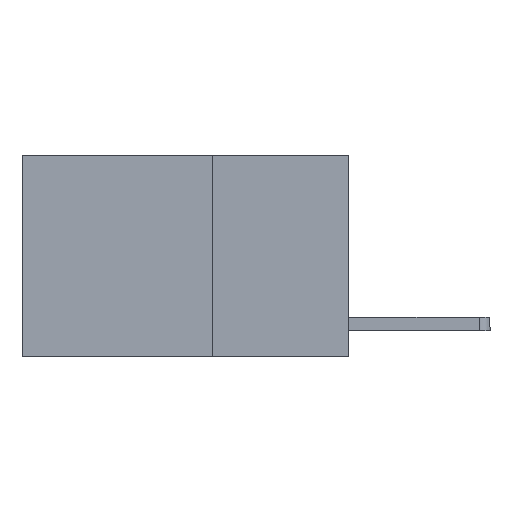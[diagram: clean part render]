
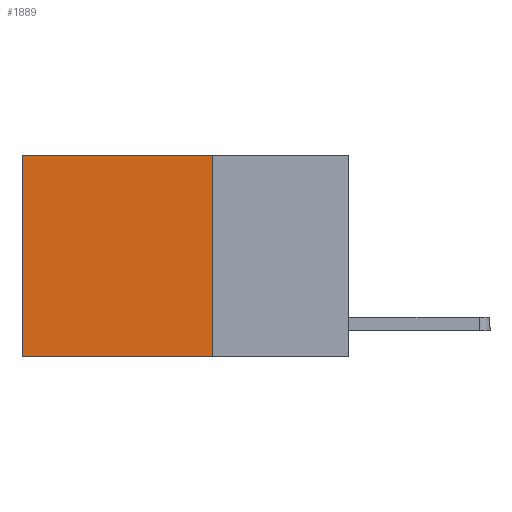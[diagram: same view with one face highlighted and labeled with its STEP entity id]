
A CAD part, left-side view. The second image highlights one B-rep face of the part: STEP entity #1889.
In plain terms, the highlighted planar face has unit normal (-1, 0, 0).
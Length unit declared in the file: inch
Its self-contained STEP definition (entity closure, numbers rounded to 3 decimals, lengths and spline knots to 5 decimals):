
#607 = LINE ( 'NONE', #1943, #8104 ) ;
#856 = VECTOR ( 'NONE', #2397, 39.37008 ) ;
#1255 = CARTESIAN_POINT ( 'NONE',  ( 0.2625, 0.25, 0. ) ) ;
#1321 = EDGE_CURVE ( 'NONE', #7605, #7886, #1727, .T. ) ;
#1387 = EDGE_LOOP ( 'NONE', ( #6431, #4426, #2238, #6048 ) ) ;
#1727 = LINE ( 'NONE', #5034, #7196 ) ;
#1889 = ADVANCED_FACE ( 'NONE', ( #4819 ), #5422, .F. ) ;
#1920 = EDGE_CURVE ( 'NONE', #1937, #4028, #2561, .T. ) ;
#1937 = VERTEX_POINT ( 'NONE', #7334 ) ;
#1943 = CARTESIAN_POINT ( 'NONE',  ( 0.2625, 0.6, 0. ) ) ;
#2156 = CARTESIAN_POINT ( 'NONE',  ( 0.2625, 0.6, -0.37 ) ) ;
#2238 = ORIENTED_EDGE ( 'NONE', *, *, #2296, .F. ) ;
#2296 = EDGE_CURVE ( 'NONE', #1937, #7605, #5830, .T. ) ;
#2397 = DIRECTION ( 'NONE',  ( 0., 0., -1. ) ) ;
#2561 = LINE ( 'NONE', #1255, #4559 ) ;
#4004 = DIRECTION ( 'NONE',  ( 0., 1., 0. ) ) ;
#4028 = VERTEX_POINT ( 'NONE', #4984 ) ;
#4086 = CARTESIAN_POINT ( 'NONE',  ( 0.2625, 0.25, 0. ) ) ;
#4395 = CARTESIAN_POINT ( 'NONE',  ( 0.2625, 0.25, -0.37 ) ) ;
#4426 = ORIENTED_EDGE ( 'NONE', *, *, #1321, .F. ) ;
#4559 = VECTOR ( 'NONE', #4004, 39.37008 ) ;
#4819 = FACE_OUTER_BOUND ( 'NONE', #1387, .T. ) ;
#4984 = CARTESIAN_POINT ( 'NONE',  ( 0.2625, 0.6, 0. ) ) ;
#4996 = EDGE_CURVE ( 'NONE', #4028, #7886, #607, .T. ) ;
#5034 = CARTESIAN_POINT ( 'NONE',  ( 0.2625, 0.25, -0.37 ) ) ;
#5121 = DIRECTION ( 'NONE',  ( 0., 1., 0. ) ) ;
#5329 = DIRECTION ( 'NONE',  ( 0., 0., -1. ) ) ;
#5422 = PLANE ( 'NONE',  #6179 ) ;
#5704 = CARTESIAN_POINT ( 'NONE',  ( 0.2625, 0.25, 0. ) ) ;
#5830 = LINE ( 'NONE', #5704, #856 ) ;
#6048 = ORIENTED_EDGE ( 'NONE', *, *, #1920, .T. ) ;
#6179 = AXIS2_PLACEMENT_3D ( 'NONE', #4086, #6753, #5329 ) ;
#6431 = ORIENTED_EDGE ( 'NONE', *, *, #4996, .T. ) ;
#6531 = DIRECTION ( 'NONE',  ( 0., 0., -1. ) ) ;
#6753 = DIRECTION ( 'NONE',  ( 1., 0., 0. ) ) ;
#7196 = VECTOR ( 'NONE', #5121, 39.37008 ) ;
#7334 = CARTESIAN_POINT ( 'NONE',  ( 0.2625, 0.25, 0. ) ) ;
#7605 = VERTEX_POINT ( 'NONE', #4395 ) ;
#7886 = VERTEX_POINT ( 'NONE', #2156 ) ;
#8104 = VECTOR ( 'NONE', #6531, 39.37008 ) ;
